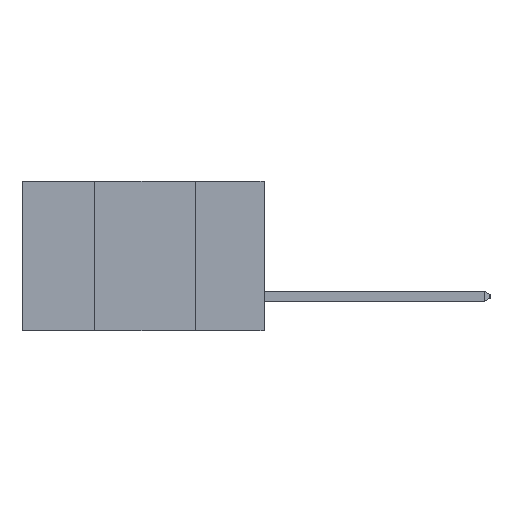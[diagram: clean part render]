
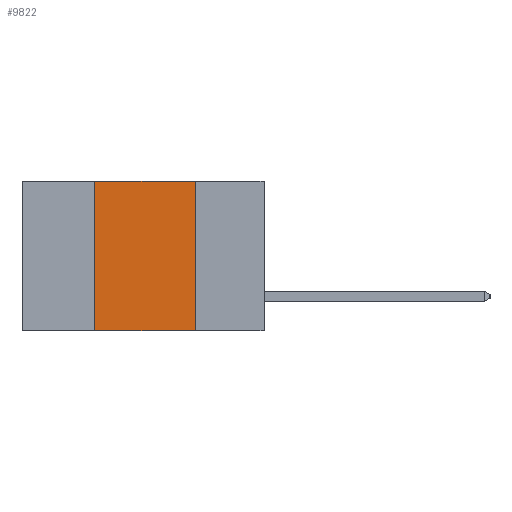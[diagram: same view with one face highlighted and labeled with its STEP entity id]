
A CAD part, left-side view. The second image highlights one B-rep face of the part: STEP entity #9822.
In plain terms, the highlighted planar face has unit normal (-1, 0, 0).
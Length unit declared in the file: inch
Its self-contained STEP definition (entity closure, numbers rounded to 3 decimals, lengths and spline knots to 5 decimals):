
#215 = ORIENTED_EDGE ( 'NONE', *, *, #15386, .F. ) ;
#2277 = DIRECTION ( 'NONE',  ( 0., -1., 0. ) ) ;
#2330 = DIRECTION ( 'NONE',  ( 0., 0., -1. ) ) ;
#2920 = VECTOR ( 'NONE', #7891, 39.37008 ) ;
#3590 = EDGE_CURVE ( 'NONE', #10379, #16611, #10552, .T. ) ;
#3821 = DIRECTION ( 'NONE',  ( 0., -1., 0. ) ) ;
#4367 = FACE_OUTER_BOUND ( 'NONE', #11759, .T. ) ;
#4386 = VECTOR ( 'NONE', #3821, 39.37008 ) ;
#4404 = ORIENTED_EDGE ( 'NONE', *, *, #3590, .F. ) ;
#4569 = VERTEX_POINT ( 'NONE', #8951 ) ;
#4838 = LINE ( 'NONE', #9550, #4386 ) ;
#4950 = CARTESIAN_POINT ( 'NONE',  ( 0., 0.17, -0.37 ) ) ;
#5408 = CARTESIAN_POINT ( 'NONE',  ( 0., 0.17, -0.37 ) ) ;
#5498 = EDGE_CURVE ( 'NONE', #10379, #17944, #4838, .T. ) ;
#6533 = CARTESIAN_POINT ( 'NONE',  ( 0., 0.42, 0. ) ) ;
#6547 = DIRECTION ( 'NONE',  ( 1., 0., 0. ) ) ;
#6888 = DIRECTION ( 'NONE',  ( 0., 0., -1. ) ) ;
#7140 = AXIS2_PLACEMENT_3D ( 'NONE', #9461, #6547, #2330 ) ;
#7891 = DIRECTION ( 'NONE',  ( 0., 0., 1. ) ) ;
#8518 = CARTESIAN_POINT ( 'NONE',  ( 0., 0.42, -0.37 ) ) ;
#8951 = CARTESIAN_POINT ( 'NONE',  ( 0., 0.17, 0. ) ) ;
#9461 = CARTESIAN_POINT ( 'NONE',  ( 0., 0.6, 0. ) ) ;
#9550 = CARTESIAN_POINT ( 'NONE',  ( 0., 0.6, -0.37 ) ) ;
#9771 = LINE ( 'NONE', #13655, #16788 ) ;
#9822 = ADVANCED_FACE ( 'NONE', ( #4367 ), #10891, .F. ) ;
#10379 = VERTEX_POINT ( 'NONE', #12119 ) ;
#10552 = LINE ( 'NONE', #8518, #2920 ) ;
#10891 = PLANE ( 'NONE',  #7140 ) ;
#10995 = LINE ( 'NONE', #5408, #15160 ) ;
#11759 = EDGE_LOOP ( 'NONE', ( #13140, #215, #4404, #15749 ) ) ;
#12119 = CARTESIAN_POINT ( 'NONE',  ( 0., 0.42, -0.37 ) ) ;
#13140 = ORIENTED_EDGE ( 'NONE', *, *, #13515, .F. ) ;
#13515 = EDGE_CURVE ( 'NONE', #4569, #17944, #10995, .T. ) ;
#13655 = CARTESIAN_POINT ( 'NONE',  ( 0., 0.6, 0. ) ) ;
#15160 = VECTOR ( 'NONE', #6888, 39.37008 ) ;
#15386 = EDGE_CURVE ( 'NONE', #16611, #4569, #9771, .T. ) ;
#15749 = ORIENTED_EDGE ( 'NONE', *, *, #5498, .T. ) ;
#16611 = VERTEX_POINT ( 'NONE', #6533 ) ;
#16788 = VECTOR ( 'NONE', #2277, 39.37008 ) ;
#17944 = VERTEX_POINT ( 'NONE', #4950 ) ;
